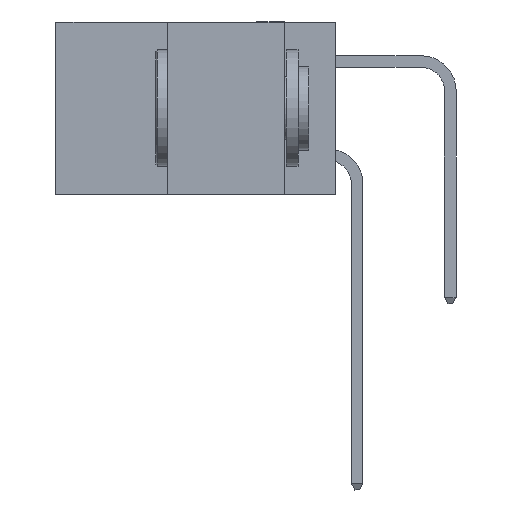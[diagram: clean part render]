
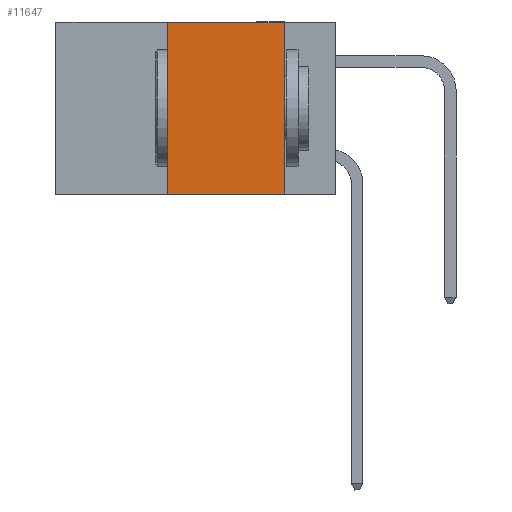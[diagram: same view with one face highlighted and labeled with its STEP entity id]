
A CAD part, left-side view. The second image highlights one B-rep face of the part: STEP entity #11647.
In plain terms, the highlighted planar face has unit normal (-1, 0, 0).
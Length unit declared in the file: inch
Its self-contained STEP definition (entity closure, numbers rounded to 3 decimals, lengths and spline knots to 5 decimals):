
#1442 = LINE ( 'NONE', #6970, #15787 ) ;
#1876 = DIRECTION ( 'NONE',  ( 0., 0., -1. ) ) ;
#1966 = EDGE_CURVE ( 'NONE', #2962, #7125, #1442, .T. ) ;
#2752 = LINE ( 'NONE', #3441, #3212 ) ;
#2784 = EDGE_CURVE ( 'NONE', #9503, #2962, #2752, .T. ) ;
#2962 = VERTEX_POINT ( 'NONE', #12497 ) ;
#3109 = DIRECTION ( 'NONE',  ( 0., -1., 0. ) ) ;
#3212 = VECTOR ( 'NONE', #3461, 39.37008 ) ;
#3441 = CARTESIAN_POINT ( 'NONE',  ( 0., 0.6, 0. ) ) ;
#3461 = DIRECTION ( 'NONE',  ( 0., -1., 0. ) ) ;
#3648 = EDGE_CURVE ( 'NONE', #6100, #7125, #17652, .T. ) ;
#6100 = VERTEX_POINT ( 'NONE', #14191 ) ;
#6411 = ORIENTED_EDGE ( 'NONE', *, *, #1966, .F. ) ;
#6731 = LINE ( 'NONE', #14109, #13653 ) ;
#6970 = CARTESIAN_POINT ( 'NONE',  ( 0., 0.11, 0. ) ) ;
#7125 = VERTEX_POINT ( 'NONE', #12605 ) ;
#7285 = ORIENTED_EDGE ( 'NONE', *, *, #12114, .F. ) ;
#7468 = DIRECTION ( 'NONE',  ( 0., 0., -1. ) ) ;
#8524 = FACE_OUTER_BOUND ( 'NONE', #15701, .T. ) ;
#8711 = CARTESIAN_POINT ( 'NONE',  ( 0., 0.6, -0.37 ) ) ;
#8984 = CARTESIAN_POINT ( 'NONE',  ( 0., 0.6, 0. ) ) ;
#9503 = VERTEX_POINT ( 'NONE', #12069 ) ;
#10119 = ORIENTED_EDGE ( 'NONE', *, *, #2784, .F. ) ;
#10353 = DIRECTION ( 'NONE',  ( 1., 0., 0. ) ) ;
#10672 = VECTOR ( 'NONE', #3109, 39.37008 ) ;
#11647 = ADVANCED_FACE ( 'NONE', ( #8524 ), #16946, .F. ) ;
#12069 = CARTESIAN_POINT ( 'NONE',  ( 0., 0.36, 0. ) ) ;
#12114 = EDGE_CURVE ( 'NONE', #6100, #9503, #6731, .T. ) ;
#12497 = CARTESIAN_POINT ( 'NONE',  ( 0., 0.11, 0. ) ) ;
#12605 = CARTESIAN_POINT ( 'NONE',  ( 0., 0.11, -0.37 ) ) ;
#12768 = AXIS2_PLACEMENT_3D ( 'NONE', #8984, #10353, #1876 ) ;
#13653 = VECTOR ( 'NONE', #15412, 39.37008 ) ;
#14109 = CARTESIAN_POINT ( 'NONE',  ( 0., 0.36, 0. ) ) ;
#14191 = CARTESIAN_POINT ( 'NONE',  ( 0., 0.36, -0.37 ) ) ;
#14996 = ORIENTED_EDGE ( 'NONE', *, *, #3648, .T. ) ;
#15412 = DIRECTION ( 'NONE',  ( 0., 0., 1. ) ) ;
#15701 = EDGE_LOOP ( 'NONE', ( #6411, #10119, #7285, #14996 ) ) ;
#15787 = VECTOR ( 'NONE', #7468, 39.37008 ) ;
#16946 = PLANE ( 'NONE',  #12768 ) ;
#17652 = LINE ( 'NONE', #8711, #10672 ) ;
